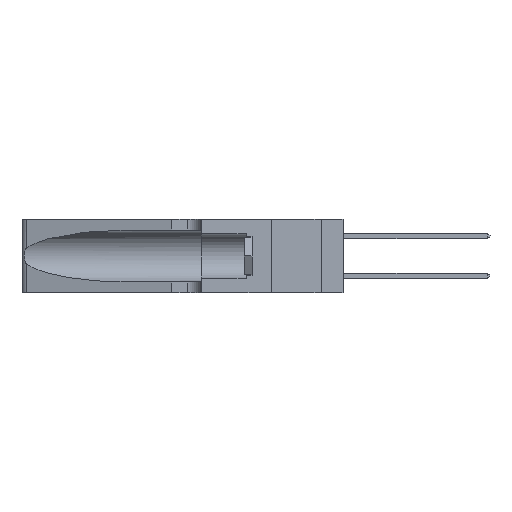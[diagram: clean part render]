
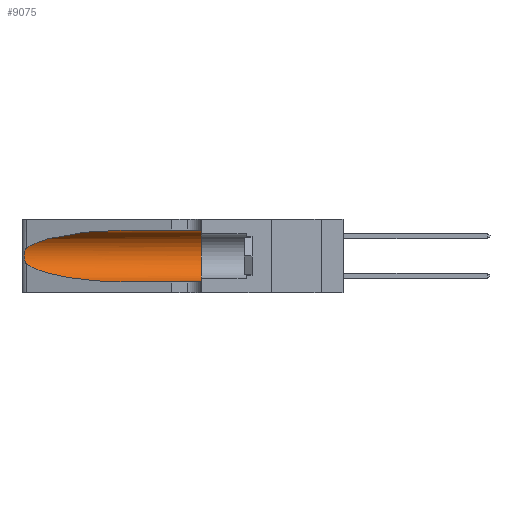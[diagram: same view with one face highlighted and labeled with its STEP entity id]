
A CAD part, left-side view. The second image highlights one B-rep face of the part: STEP entity #9075.
In plain terms, the highlighted cylindrical face has radius 3.308 mm (diameter 6.617 mm), a partial arc.
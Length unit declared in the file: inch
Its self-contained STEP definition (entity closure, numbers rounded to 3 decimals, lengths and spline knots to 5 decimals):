
#508 = CARTESIAN_POINT ( 'NONE',  ( 0.1305, 1.61858, 0.185 ) ) ;
#598 = CARTESIAN_POINT ( 'NONE',  ( 0.1305, 0.72297, 0.31525 ) ) ;
#718 = CARTESIAN_POINT ( 'NONE',  ( 0.25555, 1.22993, 0.14849 ) ) ;
#984 = B_SPLINE_CURVE_WITH_KNOTS ( 'NONE', 3,
 ( #32395, #11147, #35744, #11301, #39287, #29146, #14994, #7943, #4390, #14681, #18198, #21732, #718, #25284 ),
 .UNSPECIFIED., .F., .F.,
 ( 4, 2, 2, 2, 2, 2, 4 ),
 ( 0., 0.00027, 0.00053, 0.00107, 0.0016, 0.00187, 0.00214 ),
 .UNSPECIFIED. ) ;
#1959 = EDGE_CURVE ( 'NONE', #38566, #13581, #23579, .T. ) ;
#4020 = CARTESIAN_POINT ( 'NONE',  ( 0.1305, 1.61858, 0.31525 ) ) ;
#4237 = CARTESIAN_POINT ( 'NONE',  ( 0.25487, 1.22718, 0.14631 ) ) ;
#4317 = VECTOR ( 'NONE', #28320, 39.37008 ) ;
#4390 = CARTESIAN_POINT ( 'NONE',  ( 0.26017, 1.23833, 0.17102 ) ) ;
#4412 = VERTEX_POINT ( 'NONE', #31241 ) ;
#5474 = EDGE_LOOP ( 'NONE', ( #40495, #10623, #28124, #17320, #37982, #25400 ) ) ;
#5960 = LINE ( 'NONE', #4020, #4317 ) ;
#6215 = CARTESIAN_POINT ( 'NONE',  ( 0.2373, 1.15595, 0.08982 ) ) ;
#6582 = CARTESIAN_POINT ( 'NONE',  ( 0.1305, 0.72297, 0.05475 ) ) ;
#7844 = CYLINDRICAL_SURFACE ( 'NONE', #10667, 0.13025 ) ;
#7943 = CARTESIAN_POINT ( 'NONE',  ( 0.26075, 1.23896, 0.178 ) ) ;
#8584 = CIRCLE ( 'NONE', #34472, 0.13025 ) ;
#9075 = ADVANCED_FACE ( 'NONE', ( #41903 ), #7844, .F. ) ;
#9881 = VERTEX_POINT ( 'NONE', #4237 ) ;
#10346 = EDGE_CURVE ( 'NONE', #9881, #38566, #43779, .T. ) ;
#10623 = ORIENTED_EDGE ( 'NONE', *, *, #17298, .T. ) ;
#10667 = AXIS2_PLACEMENT_3D ( 'NONE', #508, #35232, #29258 ) ;
#11147 = CARTESIAN_POINT ( 'NONE',  ( 0.25555, 1.22994, 0.2215 ) ) ;
#11301 = CARTESIAN_POINT ( 'NONE',  ( 0.25787, 1.23484, 0.2124 ) ) ;
#13581 = VERTEX_POINT ( 'NONE', #17489 ) ;
#13600 = DIRECTION ( 'NONE',  ( 0., 0., 1. ) ) ;
#14429 = CARTESIAN_POINT ( 'NONE',  ( 0.2373, 1.15595, 0.28018 ) ) ;
#14681 = CARTESIAN_POINT ( 'NONE',  ( 0.25856, 1.23593, 0.16098 ) ) ;
#14994 = CARTESIAN_POINT ( 'NONE',  ( 0.26075, 1.23896, 0.19203 ) ) ;
#15940 = EDGE_CURVE ( 'NONE', #4412, #35854, #5960, .T. ) ;
#16776 = CARTESIAN_POINT ( 'NONE',  ( 0.1305, 0.72297, 0.05475 ) ) ;
#17093 = DIRECTION ( 'NONE',  ( 0., 1., 0. ) ) ;
#17298 = EDGE_CURVE ( 'NONE', #35238, #9881, #984, .T. ) ;
#17320 = ORIENTED_EDGE ( 'NONE', *, *, #1959, .T. ) ;
#17489 = CARTESIAN_POINT ( 'NONE',  ( 0.1305, 0.35, 0.05475 ) ) ;
#18198 = CARTESIAN_POINT ( 'NONE',  ( 0.25789, 1.23486, 0.15765 ) ) ;
#18600 = EDGE_CURVE ( 'NONE', #4412, #35238, #42381, .T. ) ;
#21462 = CARTESIAN_POINT ( 'NONE',  ( 0.25487, 1.22718, 0.22369 ) ) ;
#21732 = CARTESIAN_POINT ( 'NONE',  ( 0.25639, 1.23186, 0.15144 ) ) ;
#23579 = LINE ( 'NONE', #26513, #31893 ) ;
#25284 = CARTESIAN_POINT ( 'NONE',  ( 0.25487, 1.22718, 0.14631 ) ) ;
#25400 = ORIENTED_EDGE ( 'NONE', *, *, #15940, .F. ) ;
#26340 = CARTESIAN_POINT ( 'NONE',  ( 0.1305, 0.35, 0.31525 ) ) ;
#26513 = CARTESIAN_POINT ( 'NONE',  ( 0.1305, 1.61858, 0.05475 ) ) ;
#28124 = ORIENTED_EDGE ( 'NONE', *, *, #10346, .T. ) ;
#28320 = DIRECTION ( 'NONE',  ( 0., -1., 0. ) ) ;
#29146 = CARTESIAN_POINT ( 'NONE',  ( 0.26018, 1.23835, 0.19895 ) ) ;
#29258 = DIRECTION ( 'NONE',  ( 0., 0., -1. ) ) ;
#31241 = CARTESIAN_POINT ( 'NONE',  ( 0.1305, 0.72297, 0.31525 ) ) ;
#31597 = CARTESIAN_POINT ( 'NONE',  ( 0.1305, 0.35, 0.185 ) ) ;
#31893 = VECTOR ( 'NONE', #43700, 39.37008 ) ;
#32395 = CARTESIAN_POINT ( 'NONE',  ( 0.25487, 1.22718, 0.22369 ) ) ;
#34189 = CARTESIAN_POINT ( 'NONE',  ( 0.25487, 1.22718, 0.14631 ) ) ;
#34472 = AXIS2_PLACEMENT_3D ( 'NONE', #31597, #17093, #13600 ) ;
#35232 = DIRECTION ( 'NONE',  ( 0., -1., 0. ) ) ;
#35238 = VERTEX_POINT ( 'NONE', #43892 ) ;
#35478 = CARTESIAN_POINT ( 'NONE',  ( 0.18966, 0.96281, 0.31525 ) ) ;
#35744 = CARTESIAN_POINT ( 'NONE',  ( 0.25639, 1.23184, 0.21858 ) ) ;
#35854 = VERTEX_POINT ( 'NONE', #26340 ) ;
#37845 = CARTESIAN_POINT ( 'NONE',  ( 0.18966, 0.96281, 0.05475 ) ) ;
#37982 = ORIENTED_EDGE ( 'NONE', *, *, #39224, .F. ) ;
#38566 = VERTEX_POINT ( 'NONE', #6582 ) ;
#39224 = EDGE_CURVE ( 'NONE', #35854, #13581, #8584, .T. ) ;
#39287 = CARTESIAN_POINT ( 'NONE',  ( 0.25854, 1.2359, 0.20912 ) ) ;
#40495 = ORIENTED_EDGE ( 'NONE', *, *, #18600, .T. ) ;
#41903 = FACE_OUTER_BOUND ( 'NONE', #5474, .T. ) ;
#42381 =( BOUNDED_CURVE ( )  B_SPLINE_CURVE ( 3, ( #598, #35478, #14429, #21462 ),
 .UNSPECIFIED., .F., .F. ) 
 B_SPLINE_CURVE_WITH_KNOTS ( ( 4, 4 ),
 ( 1.5708, 2.84003 ),
 .UNSPECIFIED. ) 
 CURVE ( )  GEOMETRIC_REPRESENTATION_ITEM ( )  RATIONAL_B_SPLINE_CURVE ( ( 1., 0.87, 0.87, 1. ) ) 
 REPRESENTATION_ITEM ( '' )  );
#43700 = DIRECTION ( 'NONE',  ( 0., -1., 0. ) ) ;
#43779 =( BOUNDED_CURVE ( )  B_SPLINE_CURVE ( 3, ( #34189, #6215, #37845, #16776 ),
 .UNSPECIFIED., .F., .F. ) 
 B_SPLINE_CURVE_WITH_KNOTS ( ( 4, 4 ),
 ( 3.44316, 4.71239 ),
 .UNSPECIFIED. ) 
 CURVE ( )  GEOMETRIC_REPRESENTATION_ITEM ( )  RATIONAL_B_SPLINE_CURVE ( ( 1., 0.87, 0.87, 1. ) ) 
 REPRESENTATION_ITEM ( '' )  );
#43892 = CARTESIAN_POINT ( 'NONE',  ( 0.25487, 1.22718, 0.22369 ) ) ;
